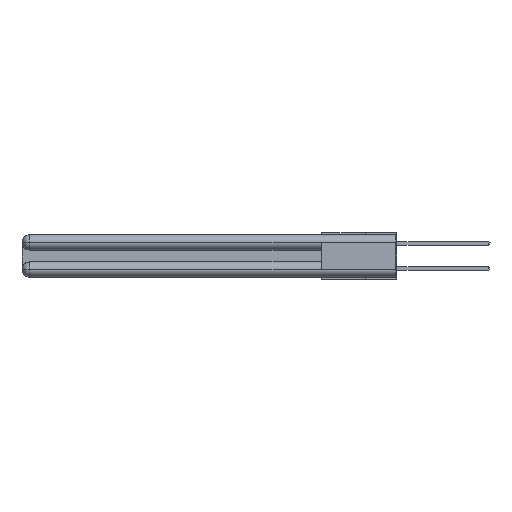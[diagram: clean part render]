
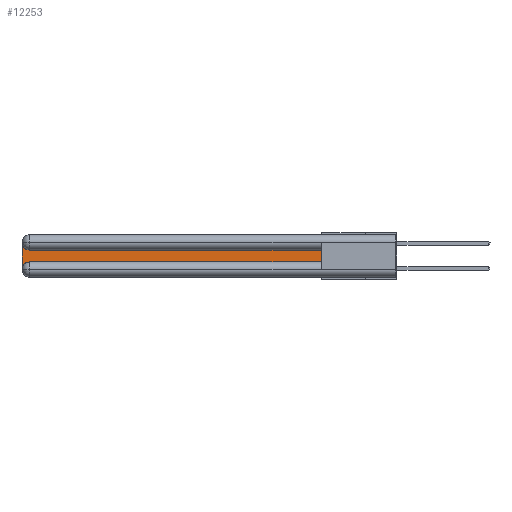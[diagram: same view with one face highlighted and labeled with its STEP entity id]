
A CAD part, left-side view. The second image highlights one B-rep face of the part: STEP entity #12253.
In plain terms, the highlighted planar face has unit normal (-1, 0, 0).
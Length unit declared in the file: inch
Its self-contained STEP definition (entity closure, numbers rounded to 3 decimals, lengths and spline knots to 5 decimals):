
#405 = EDGE_LOOP ( 'NONE', ( #22243, #3066, #12660, #939, #7672, #20283 ) ) ;
#939 = ORIENTED_EDGE ( 'NONE', *, *, #11186, .T. ) ;
#2921 = AXIS2_PLACEMENT_3D ( 'NONE', #18469, #25310, #4808 ) ;
#3066 = ORIENTED_EDGE ( 'NONE', *, *, #10087, .T. ) ;
#3955 = CARTESIAN_POINT ( 'NONE',  ( 0.075, 3., -0.2775 ) ) ;
#4808 = DIRECTION ( 'NONE',  ( 0., 0., -1. ) ) ;
#5435 = CARTESIAN_POINT ( 'NONE',  ( 0.075, 3., -0.0625 ) ) ;
#7194 = PLANE ( 'NONE',  #18399 ) ;
#7321 = CARTESIAN_POINT ( 'NONE',  ( 0.075, 0.6, -0.2175 ) ) ;
#7488 = DIRECTION ( 'NONE',  ( 1., 0., 0. ) ) ;
#7672 = ORIENTED_EDGE ( 'NONE', *, *, #9504, .T. ) ;
#8349 = EDGE_CURVE ( 'NONE', #26385, #11643, #11143, .T. ) ;
#9504 = EDGE_CURVE ( 'NONE', #16442, #23726, #25544, .T. ) ;
#9655 = DIRECTION ( 'NONE',  ( 0., 0., -1. ) ) ;
#10078 = VECTOR ( 'NONE', #16300, 39.37008 ) ;
#10087 = EDGE_CURVE ( 'NONE', #11643, #10655, #25126, .T. ) ;
#10276 = EDGE_CURVE ( 'NONE', #10655, #19549, #21940, .T. ) ;
#10440 = CARTESIAN_POINT ( 'NONE',  ( 0.075, 2.94, -0.0625 ) ) ;
#10655 = VERTEX_POINT ( 'NONE', #5435 ) ;
#11143 = LINE ( 'NONE', #13188, #13648 ) ;
#11186 = EDGE_CURVE ( 'NONE', #19549, #16442, #18308, .T. ) ;
#11643 = VERTEX_POINT ( 'NONE', #25024 ) ;
#12253 = ADVANCED_FACE ( 'NONE', ( #26393 ), #7194, .F. ) ;
#12660 = ORIENTED_EDGE ( 'NONE', *, *, #10276, .T. ) ;
#12751 = DIRECTION ( 'NONE',  ( 1., 0., 0. ) ) ;
#13188 = CARTESIAN_POINT ( 'NONE',  ( 0.075, 0.6, -0.1225 ) ) ;
#13648 = VECTOR ( 'NONE', #17805, 39.37008 ) ;
#14739 = CARTESIAN_POINT ( 'NONE',  ( 0.075, 0.6, -0.1225 ) ) ;
#14857 = EDGE_CURVE ( 'NONE', #23726, #26385, #15074, .T. ) ;
#14983 = DIRECTION ( 'NONE',  ( 0., 0., -1. ) ) ;
#15015 = DIRECTION ( 'NONE',  ( 0., 0., -1. ) ) ;
#15074 = LINE ( 'NONE', #7321, #10078 ) ;
#15484 = AXIS2_PLACEMENT_3D ( 'NONE', #10440, #12751, #15015 ) ;
#16237 = CARTESIAN_POINT ( 'NONE',  ( 0.075, 0.6, -0.2175 ) ) ;
#16300 = DIRECTION ( 'NONE',  ( 0., 0., 1. ) ) ;
#16442 = VERTEX_POINT ( 'NONE', #25789 ) ;
#16614 = VECTOR ( 'NONE', #14983, 39.37008 ) ;
#17805 = DIRECTION ( 'NONE',  ( 0., 1., 0. ) ) ;
#18308 = CIRCLE ( 'NONE', #2921, 0.06 ) ;
#18399 = AXIS2_PLACEMENT_3D ( 'NONE', #23313, #7488, #9655 ) ;
#18469 = CARTESIAN_POINT ( 'NONE',  ( 0.075, 2.94, -0.2775 ) ) ;
#19549 = VERTEX_POINT ( 'NONE', #3955 ) ;
#20283 = ORIENTED_EDGE ( 'NONE', *, *, #14857, .T. ) ;
#21281 = VECTOR ( 'NONE', #23773, 39.37008 ) ;
#21714 = CARTESIAN_POINT ( 'NONE',  ( 0.075, 0.6, -0.2175 ) ) ;
#21940 = LINE ( 'NONE', #24447, #16614 ) ;
#22243 = ORIENTED_EDGE ( 'NONE', *, *, #8349, .T. ) ;
#23313 = CARTESIAN_POINT ( 'NONE',  ( 0.075, 3., -0.1225 ) ) ;
#23726 = VERTEX_POINT ( 'NONE', #16237 ) ;
#23773 = DIRECTION ( 'NONE',  ( 0., -1., 0. ) ) ;
#24447 = CARTESIAN_POINT ( 'NONE',  ( 0.075, 3., -0.2175 ) ) ;
#25024 = CARTESIAN_POINT ( 'NONE',  ( 0.075, 2.94, -0.1225 ) ) ;
#25126 = CIRCLE ( 'NONE', #15484, 0.06 ) ;
#25310 = DIRECTION ( 'NONE',  ( 1., 0., 0. ) ) ;
#25544 = LINE ( 'NONE', #21714, #21281 ) ;
#25789 = CARTESIAN_POINT ( 'NONE',  ( 0.075, 2.94, -0.2175 ) ) ;
#26385 = VERTEX_POINT ( 'NONE', #14739 ) ;
#26393 = FACE_OUTER_BOUND ( 'NONE', #405, .T. ) ;
